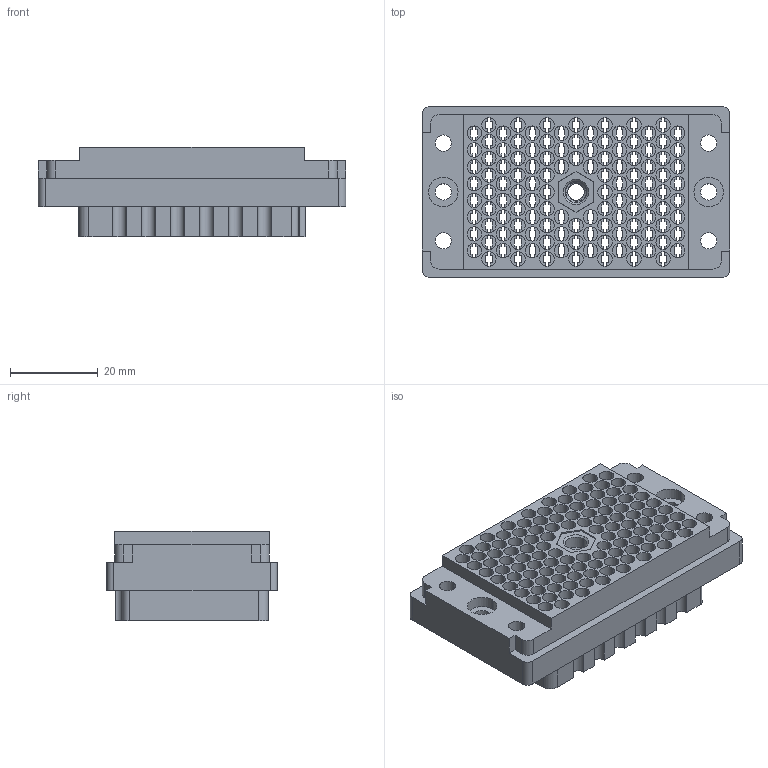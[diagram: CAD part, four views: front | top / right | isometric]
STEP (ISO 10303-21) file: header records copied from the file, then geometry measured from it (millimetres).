
FILE_DESCRIPTION (( 'STEP AP203' ), '1' );
FILE_NAME ('516-120-000-206.STEP', '2020-03-06T23:32:41', ( '' ), ( '' ), 'SwSTEP 2.0', 'SolidWorks 2016', '' );
FILE_SCHEMA (( 'CONFIG_CONTROL_DESIGN' ));
Length unit declared in the file: inch
Products named in the file (3): 516-252-095-100; 516 Part Receptacle_120; 516-120-000-206
Assembly tree (2 placements, depth 2):
  516-120-000-206
    516 Part Receptacle_120
    516-252-095-100
Bounding box: 69.85 x 38.73 x 20.27 mm (x, y, z)
Volume: 24726 mm3; surface area: 38110.6 mm2
Topology: 2 solids, 2 shells, 2537 faces, 7533 edges, 5019 vertices
Faces by surface type: plane 1802, cylinder 717, cone 12, bspline 6
Entity records: 87701 total; most frequent: CARTESIAN_POINT 17098, ORIENTED_EDGE 15066, DIRECTION 14462, EDGE_CURVE 7533, VECTOR 5580, LINE 5580, VERTEX_POINT 5019, AXIS2_PLACEMENT_3D 4441
